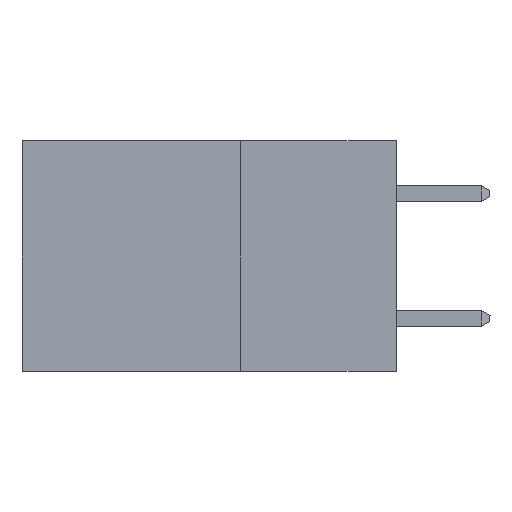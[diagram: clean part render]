
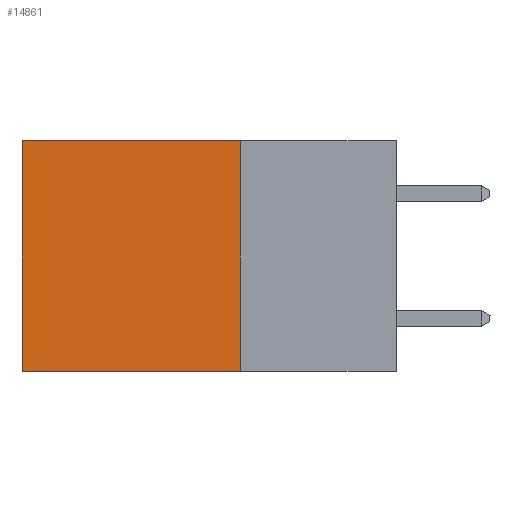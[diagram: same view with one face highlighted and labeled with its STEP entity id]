
A CAD part, left-side view. The second image highlights one B-rep face of the part: STEP entity #14861.
In plain terms, the highlighted planar face has unit normal (-1, 0, 0).
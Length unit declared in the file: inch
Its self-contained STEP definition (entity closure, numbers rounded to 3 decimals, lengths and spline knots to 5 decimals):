
#246 = EDGE_CURVE ( 'NONE', #10512, #3195, #9312, .T. ) ;
#435 = FACE_OUTER_BOUND ( 'NONE', #826, .T. ) ;
#501 = DIRECTION ( 'NONE',  ( 0., 0., -1. ) ) ;
#544 = CARTESIAN_POINT ( 'NONE',  ( 0.2615, 0.6, 0. ) ) ;
#826 = EDGE_LOOP ( 'NONE', ( #13857, #7162, #16671, #5779 ) ) ;
#2204 = PLANE ( 'NONE',  #7957 ) ;
#2452 = CARTESIAN_POINT ( 'NONE',  ( 0.2615, 0.25, -0.37 ) ) ;
#2785 = VECTOR ( 'NONE', #501, 39.37008 ) ;
#2850 = CARTESIAN_POINT ( 'NONE',  ( 0.2615, 0.25, 0. ) ) ;
#3195 = VERTEX_POINT ( 'NONE', #3609 ) ;
#3362 = EDGE_CURVE ( 'NONE', #11309, #10512, #6695, .T. ) ;
#3546 = CARTESIAN_POINT ( 'NONE',  ( 0.2615, 0.25, -0.37 ) ) ;
#3609 = CARTESIAN_POINT ( 'NONE',  ( 0.2615, 0.6, -0.37 ) ) ;
#4854 = LINE ( 'NONE', #16330, #14349 ) ;
#4884 = DIRECTION ( 'NONE',  ( 1., 0., 0. ) ) ;
#5779 = ORIENTED_EDGE ( 'NONE', *, *, #14845, .T. ) ;
#5782 = VERTEX_POINT ( 'NONE', #544 ) ;
#5841 = VECTOR ( 'NONE', #14043, 39.37008 ) ;
#6695 = LINE ( 'NONE', #12837, #13197 ) ;
#7162 = ORIENTED_EDGE ( 'NONE', *, *, #246, .F. ) ;
#7435 = DIRECTION ( 'NONE',  ( 0., 1., 0. ) ) ;
#7957 = AXIS2_PLACEMENT_3D ( 'NONE', #3546, #4884, #13953 ) ;
#9312 = LINE ( 'NONE', #9408, #5841 ) ;
#9408 = CARTESIAN_POINT ( 'NONE',  ( 0.2615, 0.25, -0.37 ) ) ;
#10244 = EDGE_CURVE ( 'NONE', #5782, #3195, #16084, .T. ) ;
#10512 = VERTEX_POINT ( 'NONE', #2452 ) ;
#11085 = CARTESIAN_POINT ( 'NONE',  ( 0.2615, 0.6, -0.37 ) ) ;
#11309 = VERTEX_POINT ( 'NONE', #2850 ) ;
#12657 = DIRECTION ( 'NONE',  ( 0., 0., -1. ) ) ;
#12837 = CARTESIAN_POINT ( 'NONE',  ( 0.2615, 0.25, -0.37 ) ) ;
#13197 = VECTOR ( 'NONE', #12657, 39.37008 ) ;
#13857 = ORIENTED_EDGE ( 'NONE', *, *, #10244, .T. ) ;
#13953 = DIRECTION ( 'NONE',  ( 0., 0., -1. ) ) ;
#14043 = DIRECTION ( 'NONE',  ( 0., 1., 0. ) ) ;
#14349 = VECTOR ( 'NONE', #7435, 39.37008 ) ;
#14845 = EDGE_CURVE ( 'NONE', #11309, #5782, #4854, .T. ) ;
#14861 = ADVANCED_FACE ( 'NONE', ( #435 ), #2204, .F. ) ;
#16084 = LINE ( 'NONE', #11085, #2785 ) ;
#16330 = CARTESIAN_POINT ( 'NONE',  ( 0.2615, 0.25, 0. ) ) ;
#16671 = ORIENTED_EDGE ( 'NONE', *, *, #3362, .F. ) ;
